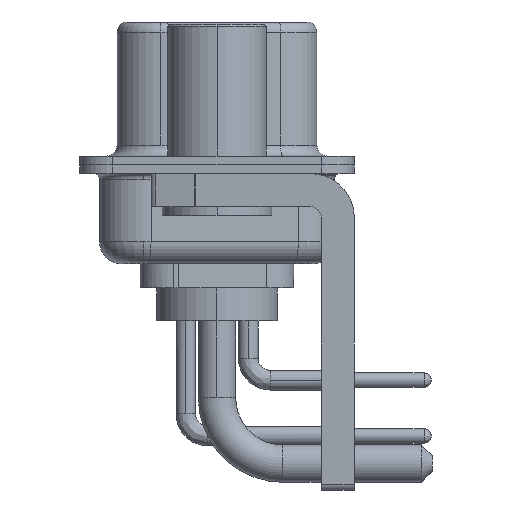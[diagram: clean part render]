
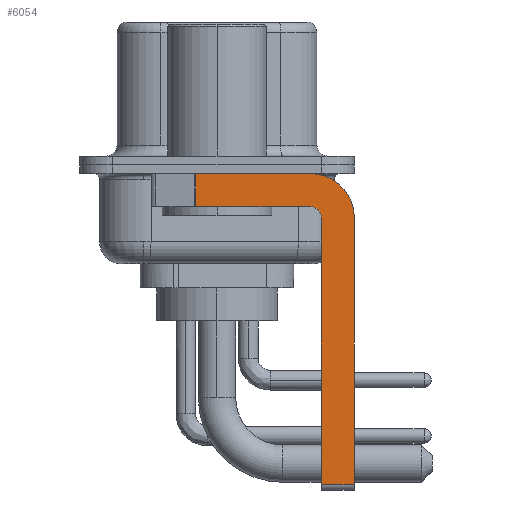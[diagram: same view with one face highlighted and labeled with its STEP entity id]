
A CAD part, left-side view. The second image highlights one B-rep face of the part: STEP entity #6054.
In plain terms, the highlighted planar face has unit normal (-1, 0, 0).
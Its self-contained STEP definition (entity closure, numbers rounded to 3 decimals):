
#110 = CARTESIAN_POINT ( 'NONE',  ( -2.9, -4.75, -14.55 ) ) ;
#402 = LINE ( 'NONE', #529, #7857 ) ;
#529 = CARTESIAN_POINT ( 'NONE',  ( -2.9, -4.25, -14.55 ) ) ;
#928 = DIRECTION ( 'NONE',  ( 0., -1., 0. ) ) ;
#1233 = ORIENTED_EDGE ( 'NONE', *, *, #10706, .F. ) ;
#1562 = DIRECTION ( 'NONE',  ( 0., 0., -1. ) ) ;
#1893 = VECTOR ( 'NONE', #2139, 1000. ) ;
#2139 = DIRECTION ( 'NONE',  ( 0., 0., -1. ) ) ;
#2255 = DIRECTION ( 'NONE',  ( 0., 0., 1. ) ) ;
#2388 = DIRECTION ( 'NONE',  ( 0., -1., 0. ) ) ;
#2626 = CARTESIAN_POINT ( 'NONE',  ( -2.9, -4.25, -1.9 ) ) ;
#3825 = VECTOR ( 'NONE', #24924, 1000. ) ;
#4066 = EDGE_CURVE ( 'NONE', #15160, #6478, #20227, .T. ) ;
#4537 = DIRECTION ( 'NONE',  ( 0., 0., -1. ) ) ;
#4598 = VERTEX_POINT ( 'NONE', #10681 ) ;
#4888 = VECTOR ( 'NONE', #2255, 1000. ) ;
#5514 = PLANE ( 'NONE',  #16823 ) ;
#5999 = ORIENTED_EDGE ( 'NONE', *, *, #4066, .T. ) ;
#6054 = ADVANCED_FACE ( 'NONE', ( #7501 ), #5514, .F. ) ;
#6478 = VERTEX_POINT ( 'NONE', #16687 ) ;
#7038 = ORIENTED_EDGE ( 'NONE', *, *, #14575, .F. ) ;
#7501 = FACE_OUTER_BOUND ( 'NONE', #13478, .T. ) ;
#7795 = ORIENTED_EDGE ( 'NONE', *, *, #21139, .T. ) ;
#7857 = VECTOR ( 'NONE', #928, 1000. ) ;
#8545 = CARTESIAN_POINT ( 'NONE',  ( -2.9, -4.75, -2.4 ) ) ;
#9639 = DIRECTION ( 'NONE',  ( -1., 0., 0. ) ) ;
#10681 = CARTESIAN_POINT ( 'NONE',  ( -2.9, -4.25, -0.4 ) ) ;
#10706 = EDGE_CURVE ( 'NONE', #15160, #4598, #12825, .T. ) ;
#12399 = CARTESIAN_POINT ( 'NONE',  ( -2.9, -6.25, -2.4 ) ) ;
#12663 = VECTOR ( 'NONE', #19702, 1000. ) ;
#12793 = LINE ( 'NONE', #16886, #3825 ) ;
#12825 = LINE ( 'NONE', #20872, #17248 ) ;
#13145 = VERTEX_POINT ( 'NONE', #22221 ) ;
#13340 = CARTESIAN_POINT ( 'NONE',  ( -2.9, -4.25, -2.4 ) ) ;
#13478 = EDGE_LOOP ( 'NONE', ( #1233, #5999, #14699, #15645, #25058, #7795, #14902, #7038 ) ) ;
#13536 = EDGE_CURVE ( 'NONE', #13145, #20225, #13627, .T. ) ;
#13573 = CARTESIAN_POINT ( 'NONE',  ( -2.9, -4.25, -2.4 ) ) ;
#13627 = LINE ( 'NONE', #12399, #12663 ) ;
#13678 = VERTEX_POINT ( 'NONE', #2626 ) ;
#13717 = EDGE_CURVE ( 'NONE', #13678, #6478, #12793, .T. ) ;
#13780 = CIRCLE ( 'NONE', #21850, 0.5 ) ;
#13845 = CARTESIAN_POINT ( 'NONE',  ( -2.9, 0.978, -0.4 ) ) ;
#14370 = AXIS2_PLACEMENT_3D ( 'NONE', #18817, #20387, #4537 ) ;
#14575 = EDGE_CURVE ( 'NONE', #4598, #13145, #24476, .T. ) ;
#14699 = ORIENTED_EDGE ( 'NONE', *, *, #13717, .F. ) ;
#14902 = ORIENTED_EDGE ( 'NONE', *, *, #13536, .F. ) ;
#15160 = VERTEX_POINT ( 'NONE', #13845 ) ;
#15191 = VERTEX_POINT ( 'NONE', #110 ) ;
#15645 = ORIENTED_EDGE ( 'NONE', *, *, #22738, .F. ) ;
#16267 = CARTESIAN_POINT ( 'NONE',  ( -2.9, 0.978, -1.9 ) ) ;
#16379 = CARTESIAN_POINT ( 'NONE',  ( -2.9, -4.75, -14.8 ) ) ;
#16687 = CARTESIAN_POINT ( 'NONE',  ( -2.9, 0.978, -1.9 ) ) ;
#16823 = AXIS2_PLACEMENT_3D ( 'NONE', #13573, #21631, #1562 ) ;
#16886 = CARTESIAN_POINT ( 'NONE',  ( -2.9, -4.25, -1.9 ) ) ;
#17248 = VECTOR ( 'NONE', #2388, 1000. ) ;
#18817 = CARTESIAN_POINT ( 'NONE',  ( -2.9, -4.25, -2.4 ) ) ;
#19552 = DIRECTION ( 'NONE',  ( 0., 0., 1. ) ) ;
#19702 = DIRECTION ( 'NONE',  ( 0., 0., -1. ) ) ;
#20225 = VERTEX_POINT ( 'NONE', #23282 ) ;
#20227 = LINE ( 'NONE', #16267, #1893 ) ;
#20387 = DIRECTION ( 'NONE',  ( 1., 0., 0. ) ) ;
#20872 = CARTESIAN_POINT ( 'NONE',  ( -2.9, 3., -0.4 ) ) ;
#21022 = EDGE_CURVE ( 'NONE', #15191, #24012, #24165, .T. ) ;
#21139 = EDGE_CURVE ( 'NONE', #15191, #20225, #402, .T. ) ;
#21631 = DIRECTION ( 'NONE',  ( 1., 0., 0. ) ) ;
#21850 = AXIS2_PLACEMENT_3D ( 'NONE', #13340, #9639, #19552 ) ;
#22221 = CARTESIAN_POINT ( 'NONE',  ( -2.9, -6.25, -2.4 ) ) ;
#22738 = EDGE_CURVE ( 'NONE', #24012, #13678, #13780, .T. ) ;
#23282 = CARTESIAN_POINT ( 'NONE',  ( -2.9, -6.25, -14.55 ) ) ;
#24012 = VERTEX_POINT ( 'NONE', #8545 ) ;
#24165 = LINE ( 'NONE', #16379, #4888 ) ;
#24476 = CIRCLE ( 'NONE', #14370, 2. ) ;
#24924 = DIRECTION ( 'NONE',  ( 0., 1., 0. ) ) ;
#25058 = ORIENTED_EDGE ( 'NONE', *, *, #21022, .F. ) ;
